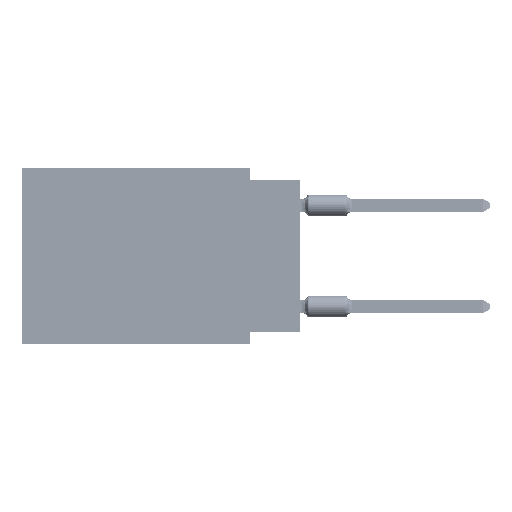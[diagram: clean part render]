
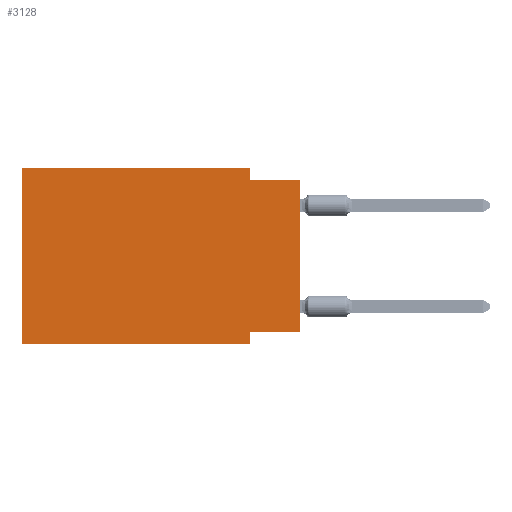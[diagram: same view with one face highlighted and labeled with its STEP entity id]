
A CAD part, left-side view. The second image highlights one B-rep face of the part: STEP entity #3128.
In plain terms, the highlighted planar face has unit normal (-1, 0, 0).
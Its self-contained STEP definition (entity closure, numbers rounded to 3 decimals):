
#1143 = DIRECTION ( 'NONE',  ( 0., -1., 0. ) ) ;
#1622 = VECTOR ( 'NONE', #70540, 1000. ) ;
#2021 = DIRECTION ( 'NONE',  ( 0., 1., 0. ) ) ;
#2023 = ORIENTED_EDGE ( 'NONE', *, *, #25576, .T. ) ;
#2303 = EDGE_CURVE ( 'NONE', #85403, #17661, #76947, .T. ) ;
#2315 = EDGE_CURVE ( 'NONE', #65838, #9692, #35291, .T. ) ;
#3128 = ADVANCED_FACE ( 'NONE', ( #9198 ), #75763, .F. ) ;
#3153 = ORIENTED_EDGE ( 'NONE', *, *, #17513, .F. ) ;
#4378 = ORIENTED_EDGE ( 'NONE', *, *, #2315, .F. ) ;
#9198 = FACE_OUTER_BOUND ( 'NONE', #77069, .T. ) ;
#9692 = VERTEX_POINT ( 'NONE', #45286 ) ;
#10190 = EDGE_CURVE ( 'NONE', #17661, #75856, #86013, .T. ) ;
#10415 = VECTOR ( 'NONE', #20710, 1000. ) ;
#11396 = VECTOR ( 'NONE', #1143, 1000. ) ;
#11413 = DIRECTION ( 'NONE',  ( 0., -1., 0. ) ) ;
#11912 = CARTESIAN_POINT ( 'NONE',  ( 0., 2.54, -8.89 ) ) ;
#17513 = EDGE_CURVE ( 'NONE', #35804, #66780, #43487, .T. ) ;
#17661 = VERTEX_POINT ( 'NONE', #87371 ) ;
#18140 = ORIENTED_EDGE ( 'NONE', *, *, #10190, .F. ) ;
#19381 = CARTESIAN_POINT ( 'NONE',  ( 0., 2.54, 0. ) ) ;
#20710 = DIRECTION ( 'NONE',  ( 0., 0., 1. ) ) ;
#25576 = EDGE_CURVE ( 'NONE', #81278, #75856, #59298, .T. ) ;
#26859 = ORIENTED_EDGE ( 'NONE', *, *, #39261, .F. ) ;
#29090 = CARTESIAN_POINT ( 'NONE',  ( 0., 2.54, 0. ) ) ;
#31363 = AXIS2_PLACEMENT_3D ( 'NONE', #82870, #43340, #49981 ) ;
#34737 = ORIENTED_EDGE ( 'NONE', *, *, #81334, .F. ) ;
#35291 = LINE ( 'NONE', #68540, #11396 ) ;
#35804 = VERTEX_POINT ( 'NONE', #59562 ) ;
#36783 = VECTOR ( 'NONE', #79637, 1000. ) ;
#38031 = CARTESIAN_POINT ( 'NONE',  ( 0., 13.97, -8.89 ) ) ;
#39261 = EDGE_CURVE ( 'NONE', #81278, #35804, #60090, .T. ) ;
#39341 = CARTESIAN_POINT ( 'NONE',  ( 0., 13.97, -8.89 ) ) ;
#40787 = CARTESIAN_POINT ( 'NONE',  ( 0., 0., -8.255 ) ) ;
#41392 = CARTESIAN_POINT ( 'NONE',  ( 0., 2.54, -0.635 ) ) ;
#43340 = DIRECTION ( 'NONE',  ( 1., 0., 0. ) ) ;
#43487 = LINE ( 'NONE', #58099, #1622 ) ;
#43827 = LINE ( 'NONE', #47320, #10415 ) ;
#45286 = CARTESIAN_POINT ( 'NONE',  ( 0., 0., -0.635 ) ) ;
#47289 = EDGE_CURVE ( 'NONE', #85403, #9692, #43827, .T. ) ;
#47320 = CARTESIAN_POINT ( 'NONE',  ( 0., 0., 0. ) ) ;
#49059 = VECTOR ( 'NONE', #11413, 1000. ) ;
#49981 = DIRECTION ( 'NONE',  ( 0., 0., -1. ) ) ;
#51990 = VECTOR ( 'NONE', #58477, 1000. ) ;
#55235 = CARTESIAN_POINT ( 'NONE',  ( 0., 2.54, -8.89 ) ) ;
#55673 = CARTESIAN_POINT ( 'NONE',  ( 0., 0., -8.255 ) ) ;
#58099 = CARTESIAN_POINT ( 'NONE',  ( 0., 13.97, 0. ) ) ;
#58477 = DIRECTION ( 'NONE',  ( 0., 0., -1. ) ) ;
#59298 = LINE ( 'NONE', #38031, #49059 ) ;
#59562 = CARTESIAN_POINT ( 'NONE',  ( 0., 13.97, 0. ) ) ;
#60090 = LINE ( 'NONE', #80509, #36783 ) ;
#63621 = ORIENTED_EDGE ( 'NONE', *, *, #47289, .T. ) ;
#65838 = VERTEX_POINT ( 'NONE', #41392 ) ;
#66780 = VERTEX_POINT ( 'NONE', #29090 ) ;
#68540 = CARTESIAN_POINT ( 'NONE',  ( 0., 0., -0.635 ) ) ;
#69662 = ORIENTED_EDGE ( 'NONE', *, *, #2303, .F. ) ;
#69873 = VECTOR ( 'NONE', #73933, 1000. ) ;
#70540 = DIRECTION ( 'NONE',  ( 0., -1., 0. ) ) ;
#73047 = LINE ( 'NONE', #19381, #69873 ) ;
#73933 = DIRECTION ( 'NONE',  ( 0., 0., -1. ) ) ;
#75763 = PLANE ( 'NONE',  #31363 ) ;
#75856 = VERTEX_POINT ( 'NONE', #55235 ) ;
#76563 = VECTOR ( 'NONE', #2021, 1000. ) ;
#76947 = LINE ( 'NONE', #55673, #76563 ) ;
#77069 = EDGE_LOOP ( 'NONE', ( #63621, #4378, #34737, #3153, #26859, #2023, #18140, #69662 ) ) ;
#79637 = DIRECTION ( 'NONE',  ( 0., 0., 1. ) ) ;
#80509 = CARTESIAN_POINT ( 'NONE',  ( 0., 13.97, 0. ) ) ;
#81278 = VERTEX_POINT ( 'NONE', #39341 ) ;
#81334 = EDGE_CURVE ( 'NONE', #66780, #65838, #73047, .T. ) ;
#82870 = CARTESIAN_POINT ( 'NONE',  ( 0., 13.97, 0. ) ) ;
#85403 = VERTEX_POINT ( 'NONE', #40787 ) ;
#86013 = LINE ( 'NONE', #11912, #51990 ) ;
#87371 = CARTESIAN_POINT ( 'NONE',  ( 0., 2.54, -8.255 ) ) ;
